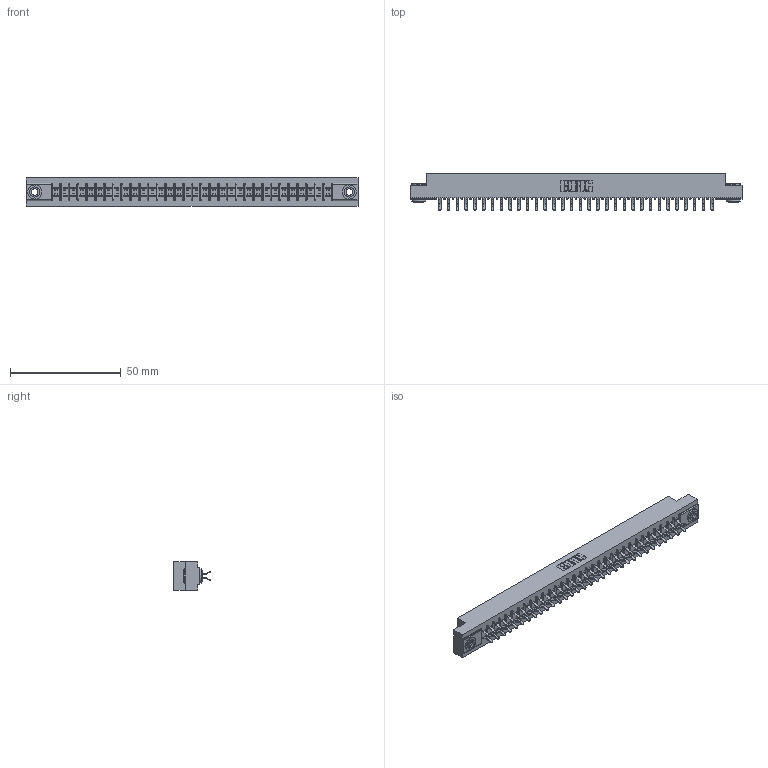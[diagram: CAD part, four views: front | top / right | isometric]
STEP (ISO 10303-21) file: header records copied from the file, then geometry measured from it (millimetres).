
FILE_DESCRIPTION (( 'STEP AP203' ), '1' );
FILE_NAME ('355-064-556-503.STEP', '2019-09-12T15:18:46', ( '' ), ( '' ), 'SwSTEP 2.0', 'SolidWorks 2016', '' );
FILE_SCHEMA (( 'CONFIG_CONTROL_DESIGN' ));
Length unit declared in the file: inch
Products named in the file (4): 355-064-556-503; 305-290-001_556; 345-250-002_345-250-002-102; 305 Part_.156 Dia
Assembly tree (67 placements, depth 2):
  355-064-556-503
    305 Part_.156 Dia
    305-290-001_556  x64
    345-250-002_345-250-002-102  x2
Bounding box: 149.81 x 16.64 x 12.7 mm (x, y, z)
Volume: 15117.1 mm3; surface area: 19985.2 mm2
Topology: 67 solids, 67 shells, 3752 faces, 10764 edges, 7000 vertices
Faces by surface type: plane 2076, cylinder 1540, sphere 128, cone 8
Entity records: 37152 total; most frequent: CARTESIAN_POINT 6131, ORIENTED_EDGE 6076, DIRECTION 5958, EDGE_CURVE 3038, LINE 2432, VECTOR 2432, VERTEX_POINT 1936, AXIS2_PLACEMENT_3D 1763
